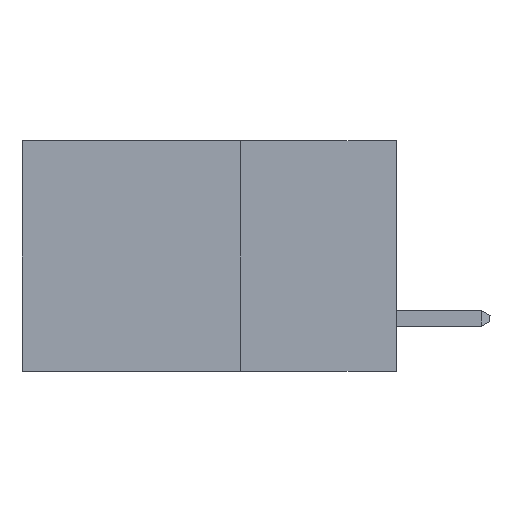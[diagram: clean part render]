
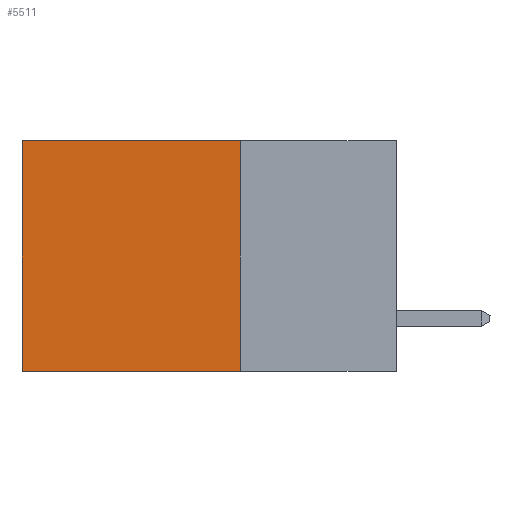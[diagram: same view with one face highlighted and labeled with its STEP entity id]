
A CAD part, left-side view. The second image highlights one B-rep face of the part: STEP entity #5511.
In plain terms, the highlighted planar face has unit normal (-1, 0, 0).
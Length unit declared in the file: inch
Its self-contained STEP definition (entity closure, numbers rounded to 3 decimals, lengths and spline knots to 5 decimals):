
#98 = CARTESIAN_POINT ( 'NONE',  ( 0.2615, 0.25, 0. ) ) ;
#318 = ORIENTED_EDGE ( 'NONE', *, *, #2570, .F. ) ;
#987 = DIRECTION ( 'NONE',  ( 0., 0., -1. ) ) ;
#1263 = CARTESIAN_POINT ( 'NONE',  ( 0.2615, 0.25, -0.37 ) ) ;
#1353 = LINE ( 'NONE', #9345, #5355 ) ;
#2141 = DIRECTION ( 'NONE',  ( 0., 0., -1. ) ) ;
#2337 = CARTESIAN_POINT ( 'NONE',  ( 0.2615, 0.25, -0.37 ) ) ;
#2570 = EDGE_CURVE ( 'NONE', #11298, #9067, #10382, .T. ) ;
#2923 = VERTEX_POINT ( 'NONE', #10102 ) ;
#3434 = ORIENTED_EDGE ( 'NONE', *, *, #11348, .F. ) ;
#3936 = AXIS2_PLACEMENT_3D ( 'NONE', #2337, #10739, #10617 ) ;
#4842 = EDGE_CURVE ( 'NONE', #13020, #2923, #1353, .T. ) ;
#5355 = VECTOR ( 'NONE', #6660, 39.37008 ) ;
#5387 = CARTESIAN_POINT ( 'NONE',  ( 0.2615, 0.25, -0.37 ) ) ;
#5511 = ADVANCED_FACE ( 'NONE', ( #8365 ), #12468, .F. ) ;
#5575 = EDGE_CURVE ( 'NONE', #2923, #9067, #5845, .T. ) ;
#5845 = LINE ( 'NONE', #9979, #8376 ) ;
#6045 = EDGE_LOOP ( 'NONE', ( #13079, #318, #3434, #8682 ) ) ;
#6660 = DIRECTION ( 'NONE',  ( 0., 1., 0. ) ) ;
#7109 = DIRECTION ( 'NONE',  ( 0., 1., 0. ) ) ;
#7184 = LINE ( 'NONE', #11259, #11345 ) ;
#8365 = FACE_OUTER_BOUND ( 'NONE', #6045, .T. ) ;
#8376 = VECTOR ( 'NONE', #987, 39.37008 ) ;
#8682 = ORIENTED_EDGE ( 'NONE', *, *, #4842, .T. ) ;
#9067 = VERTEX_POINT ( 'NONE', #9459 ) ;
#9345 = CARTESIAN_POINT ( 'NONE',  ( 0.2615, 0.25, 0. ) ) ;
#9459 = CARTESIAN_POINT ( 'NONE',  ( 0.2615, 0.6, -0.37 ) ) ;
#9979 = CARTESIAN_POINT ( 'NONE',  ( 0.2615, 0.6, -0.37 ) ) ;
#10102 = CARTESIAN_POINT ( 'NONE',  ( 0.2615, 0.6, 0. ) ) ;
#10382 = LINE ( 'NONE', #1263, #11935 ) ;
#10617 = DIRECTION ( 'NONE',  ( 0., 0., -1. ) ) ;
#10739 = DIRECTION ( 'NONE',  ( 1., 0., 0. ) ) ;
#11259 = CARTESIAN_POINT ( 'NONE',  ( 0.2615, 0.25, -0.37 ) ) ;
#11298 = VERTEX_POINT ( 'NONE', #5387 ) ;
#11345 = VECTOR ( 'NONE', #2141, 39.37008 ) ;
#11348 = EDGE_CURVE ( 'NONE', #13020, #11298, #7184, .T. ) ;
#11935 = VECTOR ( 'NONE', #7109, 39.37008 ) ;
#12468 = PLANE ( 'NONE',  #3936 ) ;
#13020 = VERTEX_POINT ( 'NONE', #98 ) ;
#13079 = ORIENTED_EDGE ( 'NONE', *, *, #5575, .T. ) ;
